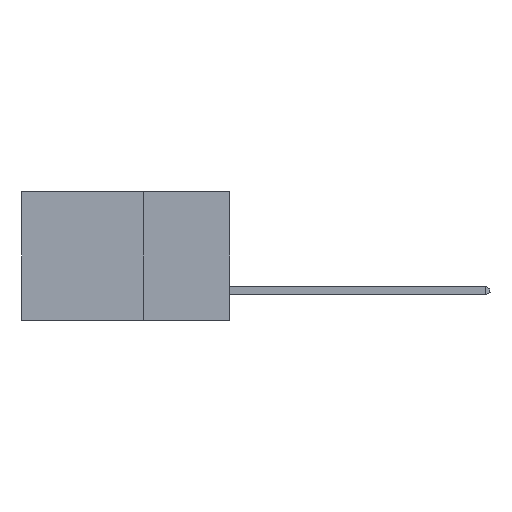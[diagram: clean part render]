
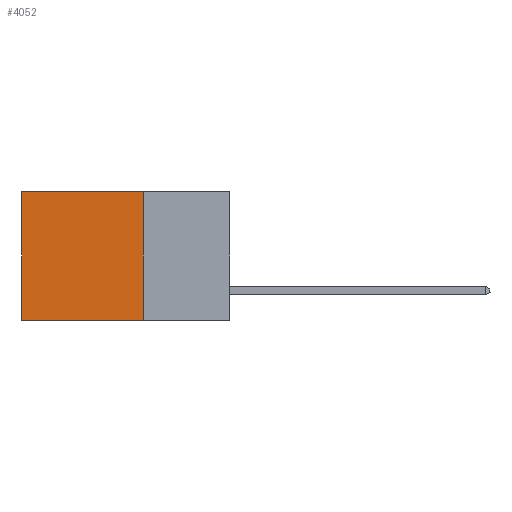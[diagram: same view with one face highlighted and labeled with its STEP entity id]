
A CAD part, left-side view. The second image highlights one B-rep face of the part: STEP entity #4052.
In plain terms, the highlighted planar face has unit normal (-1, 0, 0).
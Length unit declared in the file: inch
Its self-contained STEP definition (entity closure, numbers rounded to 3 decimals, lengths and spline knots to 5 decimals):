
#150 = EDGE_CURVE ( 'NONE', #898, #8662, #7091, .T. ) ;
#202 = ORIENTED_EDGE ( 'NONE', *, *, #657, .T. ) ;
#657 = EDGE_CURVE ( 'NONE', #8662, #17137, #4567, .T. ) ;
#849 = CARTESIAN_POINT ( 'NONE',  ( 0.298, 0.6, 0. ) ) ;
#898 = VERTEX_POINT ( 'NONE', #5148 ) ;
#2234 = CARTESIAN_POINT ( 'NONE',  ( 0.298, 0.25, 0. ) ) ;
#3462 = ORIENTED_EDGE ( 'NONE', *, *, #4147, .F. ) ;
#4052 = ADVANCED_FACE ( 'NONE', ( #7987 ), #7928, .F. ) ;
#4147 = EDGE_CURVE ( 'NONE', #898, #4165, #12110, .T. ) ;
#4165 = VERTEX_POINT ( 'NONE', #15435 ) ;
#4567 = LINE ( 'NONE', #849, #14195 ) ;
#5148 = CARTESIAN_POINT ( 'NONE',  ( 0.298, 0.25, 0. ) ) ;
#5189 = DIRECTION ( 'NONE',  ( 1., 0., 0. ) ) ;
#7091 = LINE ( 'NONE', #8829, #17865 ) ;
#7921 = ORIENTED_EDGE ( 'NONE', *, *, #150, .T. ) ;
#7928 = PLANE ( 'NONE',  #17947 ) ;
#7987 = FACE_OUTER_BOUND ( 'NONE', #11123, .T. ) ;
#8004 = CARTESIAN_POINT ( 'NONE',  ( 0.298, 0.25, 0. ) ) ;
#8150 = DIRECTION ( 'NONE',  ( 0., 0., -1. ) ) ;
#8662 = VERTEX_POINT ( 'NONE', #14528 ) ;
#8829 = CARTESIAN_POINT ( 'NONE',  ( 0.298, 0.25, 0. ) ) ;
#9265 = EDGE_CURVE ( 'NONE', #4165, #17137, #11076, .T. ) ;
#9516 = CARTESIAN_POINT ( 'NONE',  ( 0.298, 0.25, -0.37 ) ) ;
#9656 = DIRECTION ( 'NONE',  ( 0., 1., 0. ) ) ;
#10154 = VECTOR ( 'NONE', #9656, 39.37008 ) ;
#11076 = LINE ( 'NONE', #9516, #10154 ) ;
#11123 = EDGE_LOOP ( 'NONE', ( #202, #16344, #3462, #7921 ) ) ;
#11871 = VECTOR ( 'NONE', #16894, 39.37008 ) ;
#12110 = LINE ( 'NONE', #8004, #11871 ) ;
#14195 = VECTOR ( 'NONE', #8150, 39.37008 ) ;
#14528 = CARTESIAN_POINT ( 'NONE',  ( 0.298, 0.6, 0. ) ) ;
#15435 = CARTESIAN_POINT ( 'NONE',  ( 0.298, 0.25, -0.37 ) ) ;
#16344 = ORIENTED_EDGE ( 'NONE', *, *, #9265, .F. ) ;
#16690 = DIRECTION ( 'NONE',  ( 0., 0., -1. ) ) ;
#16894 = DIRECTION ( 'NONE',  ( 0., 0., -1. ) ) ;
#17137 = VERTEX_POINT ( 'NONE', #18634 ) ;
#17518 = DIRECTION ( 'NONE',  ( 0., 1., 0. ) ) ;
#17865 = VECTOR ( 'NONE', #17518, 39.37008 ) ;
#17947 = AXIS2_PLACEMENT_3D ( 'NONE', #2234, #5189, #16690 ) ;
#18634 = CARTESIAN_POINT ( 'NONE',  ( 0.298, 0.6, -0.37 ) ) ;
